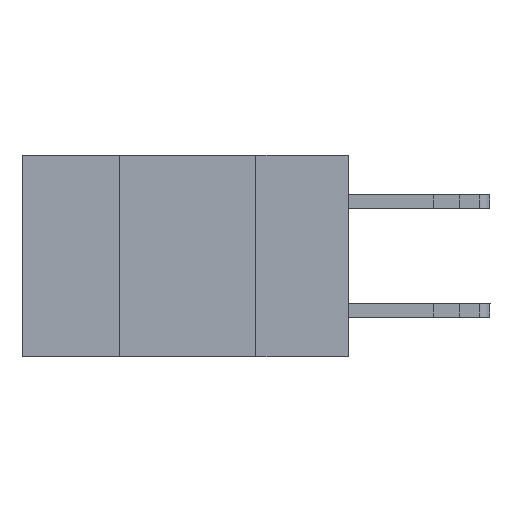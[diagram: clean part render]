
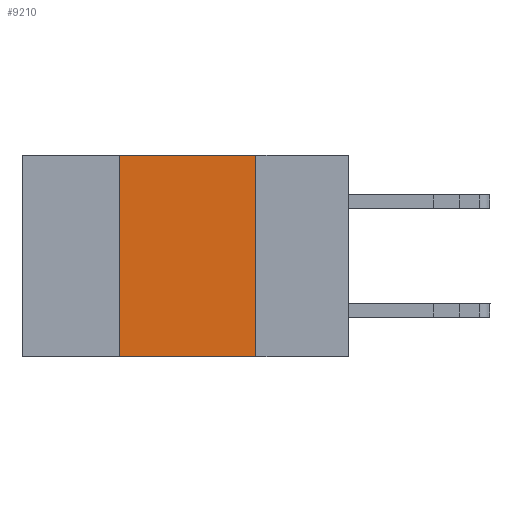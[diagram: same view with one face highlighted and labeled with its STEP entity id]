
A CAD part, left-side view. The second image highlights one B-rep face of the part: STEP entity #9210.
In plain terms, the highlighted planar face has unit normal (-1, 0, 0).
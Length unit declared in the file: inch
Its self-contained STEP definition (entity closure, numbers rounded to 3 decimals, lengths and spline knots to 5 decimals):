
#62 = AXIS2_PLACEMENT_3D ( 'NONE', #1977, #8399, #2937 ) ;
#421 = CARTESIAN_POINT ( 'NONE',  ( 0., 0.42, 0. ) ) ;
#614 = VERTEX_POINT ( 'NONE', #421 ) ;
#1977 = CARTESIAN_POINT ( 'NONE',  ( 0., 0.6, 0. ) ) ;
#2574 = DIRECTION ( 'NONE',  ( 0., -1., 0. ) ) ;
#2937 = DIRECTION ( 'NONE',  ( 0., 0., -1. ) ) ;
#3000 = ORIENTED_EDGE ( 'NONE', *, *, #10497, .T. ) ;
#3724 = CARTESIAN_POINT ( 'NONE',  ( 0., 0.42, -0.37 ) ) ;
#3893 = CARTESIAN_POINT ( 'NONE',  ( 0., 0.17, 0. ) ) ;
#4403 = LINE ( 'NONE', #11214, #6900 ) ;
#4420 = VERTEX_POINT ( 'NONE', #11192 ) ;
#4707 = DIRECTION ( 'NONE',  ( 0., 0., 1. ) ) ;
#5089 = ORIENTED_EDGE ( 'NONE', *, *, #9481, .F. ) ;
#5092 = CARTESIAN_POINT ( 'NONE',  ( 0., 0.42, -0.37 ) ) ;
#5137 = ORIENTED_EDGE ( 'NONE', *, *, #9877, .F. ) ;
#6530 = CARTESIAN_POINT ( 'NONE',  ( 0., 0.17, -0.37 ) ) ;
#6630 = LINE ( 'NONE', #6530, #10868 ) ;
#6708 = PLANE ( 'NONE',  #62 ) ;
#6900 = VECTOR ( 'NONE', #8703, 39.37008 ) ;
#6990 = VERTEX_POINT ( 'NONE', #5092 ) ;
#7388 = DIRECTION ( 'NONE',  ( 0., 0., -1. ) ) ;
#8399 = DIRECTION ( 'NONE',  ( 1., 0., 0. ) ) ;
#8703 = DIRECTION ( 'NONE',  ( 0., -1., 0. ) ) ;
#8950 = CARTESIAN_POINT ( 'NONE',  ( 0., 0.6, -0.37 ) ) ;
#9036 = EDGE_CURVE ( 'NONE', #9999, #4420, #6630, .T. ) ;
#9210 = ADVANCED_FACE ( 'NONE', ( #9296 ), #6708, .F. ) ;
#9296 = FACE_OUTER_BOUND ( 'NONE', #10278, .T. ) ;
#9481 = EDGE_CURVE ( 'NONE', #614, #9999, #4403, .T. ) ;
#9877 = EDGE_CURVE ( 'NONE', #6990, #614, #11566, .T. ) ;
#9961 = ORIENTED_EDGE ( 'NONE', *, *, #9036, .F. ) ;
#9992 = VECTOR ( 'NONE', #2574, 39.37008 ) ;
#9999 = VERTEX_POINT ( 'NONE', #3893 ) ;
#10278 = EDGE_LOOP ( 'NONE', ( #9961, #5089, #5137, #3000 ) ) ;
#10497 = EDGE_CURVE ( 'NONE', #6990, #4420, #11080, .T. ) ;
#10868 = VECTOR ( 'NONE', #7388, 39.37008 ) ;
#11080 = LINE ( 'NONE', #8950, #9992 ) ;
#11192 = CARTESIAN_POINT ( 'NONE',  ( 0., 0.17, -0.37 ) ) ;
#11214 = CARTESIAN_POINT ( 'NONE',  ( 0., 0.6, 0. ) ) ;
#11328 = VECTOR ( 'NONE', #4707, 39.37008 ) ;
#11566 = LINE ( 'NONE', #3724, #11328 ) ;
